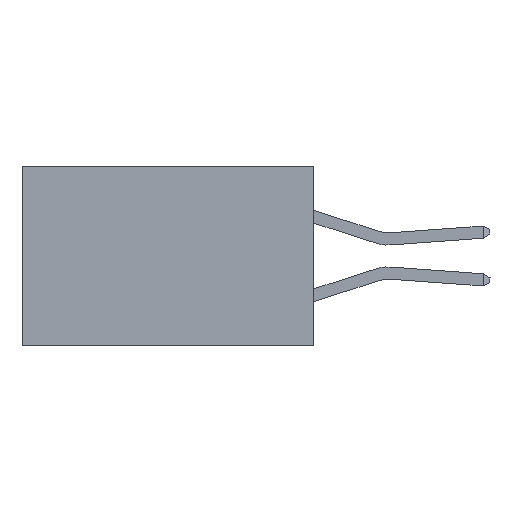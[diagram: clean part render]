
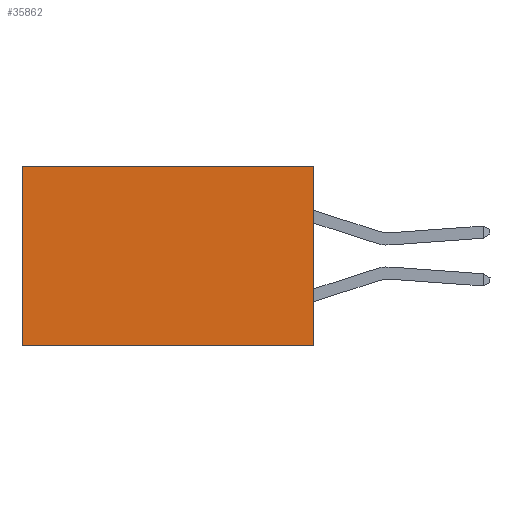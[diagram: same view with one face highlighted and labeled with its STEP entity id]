
A CAD part, left-side view. The second image highlights one B-rep face of the part: STEP entity #35862.
In plain terms, the highlighted planar face has unit normal (-1, 0, 0).
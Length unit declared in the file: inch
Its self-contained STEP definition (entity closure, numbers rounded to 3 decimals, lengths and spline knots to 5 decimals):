
#1170 = DIRECTION ( 'NONE',  ( 0., 0., -1. ) ) ;
#1833 = VECTOR ( 'NONE', #2130, 39.37008 ) ;
#1845 = EDGE_LOOP ( 'NONE', ( #9454, #12034, #4908, #14944 ) ) ;
#2130 = DIRECTION ( 'NONE',  ( 0., 1., 0. ) ) ;
#2648 = CARTESIAN_POINT ( 'NONE',  ( 0.2875, 0., 0. ) ) ;
#3478 = DIRECTION ( 'NONE',  ( 0., 1., 0. ) ) ;
#3550 = VECTOR ( 'NONE', #3478, 39.37008 ) ;
#4330 = AXIS2_PLACEMENT_3D ( 'NONE', #23381, #20366, #1170 ) ;
#4908 = ORIENTED_EDGE ( 'NONE', *, *, #23674, .F. ) ;
#6737 = VECTOR ( 'NONE', #15958, 39.37008 ) ;
#7172 = CARTESIAN_POINT ( 'NONE',  ( 0.2875, 0.6, 0. ) ) ;
#9454 = ORIENTED_EDGE ( 'NONE', *, *, #39832, .T. ) ;
#10362 = VERTEX_POINT ( 'NONE', #2648 ) ;
#10433 = DIRECTION ( 'NONE',  ( 0., 0., -1. ) ) ;
#12034 = ORIENTED_EDGE ( 'NONE', *, *, #36615, .F. ) ;
#12117 = LINE ( 'NONE', #19413, #3550 ) ;
#12763 = CARTESIAN_POINT ( 'NONE',  ( 0.2875, 0., 0. ) ) ;
#14001 = FACE_OUTER_BOUND ( 'NONE', #1845, .T. ) ;
#14944 = ORIENTED_EDGE ( 'NONE', *, *, #34539, .T. ) ;
#15958 = DIRECTION ( 'NONE',  ( 0., 0., -1. ) ) ;
#16246 = LINE ( 'NONE', #12763, #6737 ) ;
#17200 = PLANE ( 'NONE',  #4330 ) ;
#18109 = CARTESIAN_POINT ( 'NONE',  ( 0.2875, 0., -0.37 ) ) ;
#19413 = CARTESIAN_POINT ( 'NONE',  ( 0.2875, 0., 0. ) ) ;
#20366 = DIRECTION ( 'NONE',  ( 1., 0., 0. ) ) ;
#23381 = CARTESIAN_POINT ( 'NONE',  ( 0.2875, 0., 0. ) ) ;
#23674 = EDGE_CURVE ( 'NONE', #10362, #30673, #16246, .T. ) ;
#27543 = VERTEX_POINT ( 'NONE', #39175 ) ;
#28674 = VECTOR ( 'NONE', #10433, 39.37008 ) ;
#29102 = CARTESIAN_POINT ( 'NONE',  ( 0.2875, 0.6, 0. ) ) ;
#30356 = VERTEX_POINT ( 'NONE', #29102 ) ;
#30673 = VERTEX_POINT ( 'NONE', #40403 ) ;
#34539 = EDGE_CURVE ( 'NONE', #10362, #30356, #12117, .T. ) ;
#34691 = LINE ( 'NONE', #18109, #1833 ) ;
#35862 = ADVANCED_FACE ( 'NONE', ( #14001 ), #17200, .F. ) ;
#36615 = EDGE_CURVE ( 'NONE', #30673, #27543, #34691, .T. ) ;
#39116 = LINE ( 'NONE', #7172, #28674 ) ;
#39175 = CARTESIAN_POINT ( 'NONE',  ( 0.2875, 0.6, -0.37 ) ) ;
#39832 = EDGE_CURVE ( 'NONE', #30356, #27543, #39116, .T. ) ;
#40403 = CARTESIAN_POINT ( 'NONE',  ( 0.2875, 0., -0.37 ) ) ;
